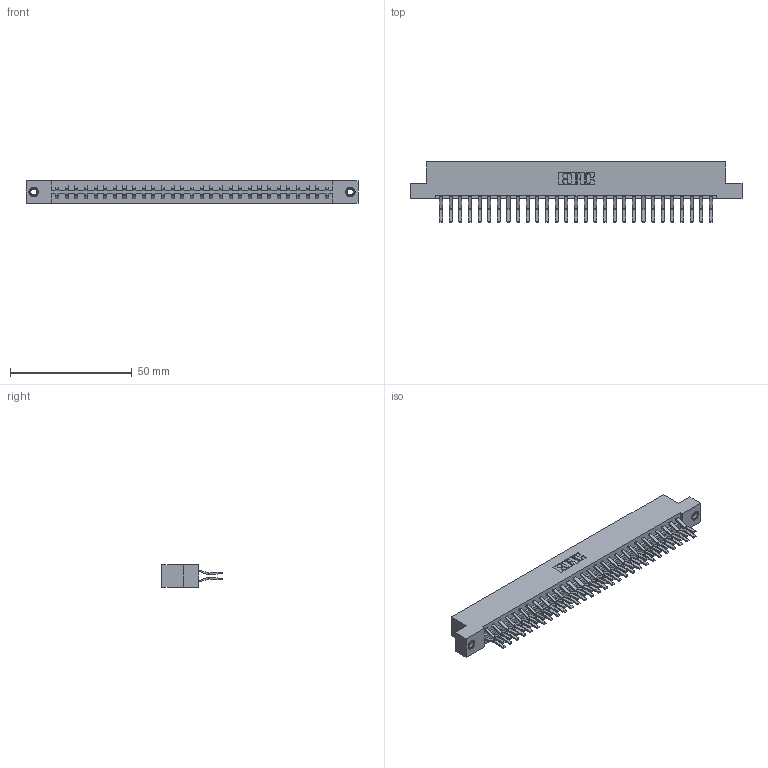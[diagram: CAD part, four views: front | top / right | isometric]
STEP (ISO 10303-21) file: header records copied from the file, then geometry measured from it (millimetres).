
FILE_DESCRIPTION (( 'STEP AP203' ), '1' );
FILE_NAME ('333-058-560-207.STEP', '2018-08-04T06:38:40', ( '' ), ( '' ), 'SwSTEP 2.0', 'SolidWorks 2016', '' );
FILE_SCHEMA (( 'CONFIG_CONTROL_DESIGN' ));
Length unit declared in the file: inch
Products named in the file (4): 345-250-001_345-250-005-103; 333-058-560-207; 333 Part_Flush - .156 Dia - TI; 345-292-001_560 Tail
Assembly tree (61 placements, depth 2):
  333-058-560-207
    333 Part_Flush - .156 Dia - TI
    345-292-001_560 Tail  x58
    345-250-001_345-250-005-103  x2
Bounding box: 136.45 x 24.78 x 9.4 mm (x, y, z)
Volume: 14175.7 mm3; surface area: 17738.2 mm2
Topology: 61 solids, 61 shells, 3306 faces, 9785 edges, 6438 vertices
Faces by surface type: plane 2190, cylinder 1100, cone 12, torus 4
Entity records: 21612 total; most frequent: CARTESIAN_POINT 3581, ORIENTED_EDGE 3510, DIRECTION 3117, EDGE_CURVE 1755, LINE 1603, VECTOR 1603, VERTEX_POINT 1164, AXIS2_PLACEMENT_3D 757
